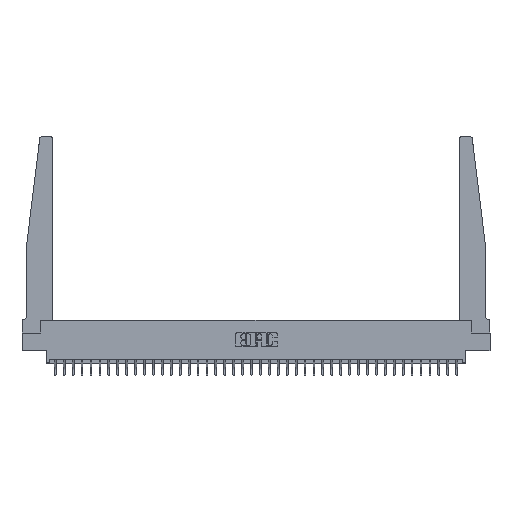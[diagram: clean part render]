
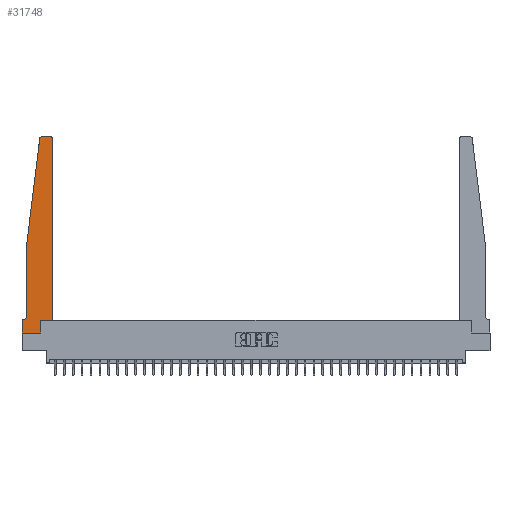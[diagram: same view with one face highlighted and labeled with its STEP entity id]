
A CAD part, top view. The second image highlights one B-rep face of the part: STEP entity #31748.
In plain terms, the highlighted planar face has unit normal (0, 0, 1).
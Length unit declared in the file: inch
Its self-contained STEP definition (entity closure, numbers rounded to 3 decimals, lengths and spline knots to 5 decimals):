
#67 = DIRECTION ( 'NONE',  ( 0., 0., 1. ) ) ;
#528 = VERTEX_POINT ( 'NONE', #5007 ) ;
#725 = CARTESIAN_POINT ( 'NONE',  ( 0.065, 0.2375, 0.37 ) ) ;
#1007 = DIRECTION ( 'NONE',  ( 0., -1., 0. ) ) ;
#2030 = ORIENTED_EDGE ( 'NONE', *, *, #10077, .T. ) ;
#2631 = VERTEX_POINT ( 'NONE', #725 ) ;
#2640 = VECTOR ( 'NONE', #1007, 39.37008 ) ;
#2778 = DIRECTION ( 'NONE',  ( 0., 0., -1. ) ) ;
#3028 = EDGE_CURVE ( 'NONE', #4124, #26963, #29324, .T. ) ;
#3127 = VECTOR ( 'NONE', #14454, 39.37008 ) ;
#3494 = LINE ( 'NONE', #19946, #2640 ) ;
#3542 = CARTESIAN_POINT ( 'NONE',  ( 0.27653, 2.72, 0.37 ) ) ;
#4124 = VERTEX_POINT ( 'NONE', #23718 ) ;
#4164 = ORIENTED_EDGE ( 'NONE', *, *, #18975, .T. ) ;
#4481 = VECTOR ( 'NONE', #12872, 39.37008 ) ;
#4865 = CARTESIAN_POINT ( 'NONE',  ( 0.425, 2.72, 0.37 ) ) ;
#5007 = CARTESIAN_POINT ( 'NONE',  ( 0., 0.1875, 0.37 ) ) ;
#5064 = DIRECTION ( 'NONE',  ( 0., -1., 0. ) ) ;
#5184 = VECTOR ( 'NONE', #30541, 39.37008 ) ;
#5293 = CARTESIAN_POINT ( 'NONE',  ( 0.015, 0.1875, 0.37 ) ) ;
#5635 = CARTESIAN_POINT ( 'NONE',  ( 0.425, 0.18, 0.37 ) ) ;
#6027 = VERTEX_POINT ( 'NONE', #22489 ) ;
#6119 = CARTESIAN_POINT ( 'NONE',  ( 0.2605, 0.18, 0.37 ) ) ;
#6296 = DIRECTION ( 'NONE',  ( 1., 0., 0. ) ) ;
#6726 = ORIENTED_EDGE ( 'NONE', *, *, #7844, .T. ) ;
#7589 = EDGE_CURVE ( 'NONE', #21215, #4124, #32333, .T. ) ;
#7811 = CARTESIAN_POINT ( 'NONE',  ( 0.065, 1.25, 0.37 ) ) ;
#7844 = EDGE_CURVE ( 'NONE', #528, #31717, #3494, .T. ) ;
#8389 = DIRECTION ( 'NONE',  ( 1., 0., 0. ) ) ;
#8815 = VECTOR ( 'NONE', #8389, 39.37008 ) ;
#9297 = ORIENTED_EDGE ( 'NONE', *, *, #11489, .T. ) ;
#9444 = PLANE ( 'NONE',  #27056 ) ;
#9688 = EDGE_CURVE ( 'NONE', #26963, #18637, #15705, .T. ) ;
#10077 = EDGE_CURVE ( 'NONE', #6027, #2631, #18207, .T. ) ;
#10112 = ORIENTED_EDGE ( 'NONE', *, *, #9688, .T. ) ;
#10209 = EDGE_LOOP ( 'NONE', ( #24317, #10112, #9297, #2030, #22724, #21066, #6726, #18561, #4164, #30090, #34571, #20601 ) ) ;
#11489 = EDGE_CURVE ( 'NONE', #18637, #6027, #33758, .T. ) ;
#12085 = LINE ( 'NONE', #19870, #3127 ) ;
#12145 = DIRECTION ( 'NONE',  ( 0., 0., 1. ) ) ;
#12872 = DIRECTION ( 'NONE',  ( -1., 0., 0. ) ) ;
#14005 = EDGE_CURVE ( 'NONE', #23192, #21215, #12085, .T. ) ;
#14454 = DIRECTION ( 'NONE',  ( 0., 1., 0. ) ) ;
#14543 = CARTESIAN_POINT ( 'NONE',  ( 0., 0., 0.37 ) ) ;
#15163 = CARTESIAN_POINT ( 'NONE',  ( 0.2605, 0., 0.37 ) ) ;
#15474 = CARTESIAN_POINT ( 'NONE',  ( 0.425, 0.18, 0.37 ) ) ;
#15544 = DIRECTION ( 'NONE',  ( -1., 0., 0. ) ) ;
#15705 = CIRCLE ( 'NONE', #33388, 0.03 ) ;
#16103 = VECTOR ( 'NONE', #15544, 39.37008 ) ;
#16344 = CARTESIAN_POINT ( 'NONE',  ( 0.395, 2.72, 0.37 ) ) ;
#16858 = CARTESIAN_POINT ( 'NONE',  ( 0.2605, 0.18, 0.37 ) ) ;
#18207 = LINE ( 'NONE', #7811, #31375 ) ;
#18561 = ORIENTED_EDGE ( 'NONE', *, *, #33113, .T. ) ;
#18637 = VERTEX_POINT ( 'NONE', #28926 ) ;
#18883 = LINE ( 'NONE', #28682, #4481 ) ;
#18975 = EDGE_CURVE ( 'NONE', #19804, #21475, #21946, .T. ) ;
#19022 = CARTESIAN_POINT ( 'NONE',  ( 0.015, 0.2375, 0.37 ) ) ;
#19043 = DIRECTION ( 'NONE',  ( 1., 0., 0. ) ) ;
#19045 = AXIS2_PLACEMENT_3D ( 'NONE', #16344, #67, #19043 ) ;
#19773 = VECTOR ( 'NONE', #22805, 39.37008 ) ;
#19804 = VERTEX_POINT ( 'NONE', #15163 ) ;
#19870 = CARTESIAN_POINT ( 'NONE',  ( 0.425, 0.18, 0.37 ) ) ;
#19946 = CARTESIAN_POINT ( 'NONE',  ( 0., 0., 0.37 ) ) ;
#20601 = ORIENTED_EDGE ( 'NONE', *, *, #7589, .T. ) ;
#20924 = CARTESIAN_POINT ( 'NONE',  ( 0.25, 2.75, 0.37 ) ) ;
#21066 = ORIENTED_EDGE ( 'NONE', *, *, #31259, .T. ) ;
#21215 = VERTEX_POINT ( 'NONE', #4865 ) ;
#21475 = VERTEX_POINT ( 'NONE', #16858 ) ;
#21687 = DIRECTION ( 'NONE',  ( -1., 0., 0. ) ) ;
#21946 = LINE ( 'NONE', #6119, #28096 ) ;
#22412 = DIRECTION ( 'NONE',  ( 0., 0., 1. ) ) ;
#22489 = CARTESIAN_POINT ( 'NONE',  ( 0.065, 1.25, 0.37 ) ) ;
#22724 = ORIENTED_EDGE ( 'NONE', *, *, #29507, .T. ) ;
#22805 = DIRECTION ( 'NONE',  ( -0.122, -0.992, 0. ) ) ;
#23192 = VERTEX_POINT ( 'NONE', #15474 ) ;
#23634 = AXIS2_PLACEMENT_3D ( 'NONE', #19022, #2778, #21687 ) ;
#23718 = CARTESIAN_POINT ( 'NONE',  ( 0.395, 2.75, 0.37 ) ) ;
#24317 = ORIENTED_EDGE ( 'NONE', *, *, #3028, .T. ) ;
#26574 = LINE ( 'NONE', #14543, #5184 ) ;
#26963 = VERTEX_POINT ( 'NONE', #33178 ) ;
#27056 = AXIS2_PLACEMENT_3D ( 'NONE', #28080, #12145, #30721 ) ;
#27350 = VERTEX_POINT ( 'NONE', #5293 ) ;
#27522 = DIRECTION ( 'NONE',  ( 0., 1., 0. ) ) ;
#28080 = CARTESIAN_POINT ( 'NONE',  ( 0., 0.1875, 0.37 ) ) ;
#28096 = VECTOR ( 'NONE', #27522, 39.37008 ) ;
#28682 = CARTESIAN_POINT ( 'NONE',  ( 0.065, 0.1875, 0.37 ) ) ;
#28926 = CARTESIAN_POINT ( 'NONE',  ( 0.24675, 2.72367, 0.37 ) ) ;
#29324 = LINE ( 'NONE', #20924, #16103 ) ;
#29507 = EDGE_CURVE ( 'NONE', #2631, #27350, #30891, .T. ) ;
#29561 = EDGE_CURVE ( 'NONE', #21475, #23192, #30059, .T. ) ;
#30059 = LINE ( 'NONE', #5635, #8815 ) ;
#30090 = ORIENTED_EDGE ( 'NONE', *, *, #29561, .T. ) ;
#30541 = DIRECTION ( 'NONE',  ( 1., 0., 0. ) ) ;
#30712 = CARTESIAN_POINT ( 'NONE',  ( 0.065, 1.25, 0.37 ) ) ;
#30721 = DIRECTION ( 'NONE',  ( 1., 0., 0. ) ) ;
#30891 = CIRCLE ( 'NONE', #23634, 0.05 ) ;
#31259 = EDGE_CURVE ( 'NONE', #27350, #528, #18883, .T. ) ;
#31375 = VECTOR ( 'NONE', #5064, 39.37008 ) ;
#31717 = VERTEX_POINT ( 'NONE', #33240 ) ;
#31748 = ADVANCED_FACE ( 'NONE', ( #32824 ), #9444, .T. ) ;
#32333 = CIRCLE ( 'NONE', #19045, 0.03 ) ;
#32824 = FACE_OUTER_BOUND ( 'NONE', #10209, .T. ) ;
#33113 = EDGE_CURVE ( 'NONE', #31717, #19804, #26574, .T. ) ;
#33178 = CARTESIAN_POINT ( 'NONE',  ( 0.27653, 2.75, 0.37 ) ) ;
#33240 = CARTESIAN_POINT ( 'NONE',  ( 0., 0., 0.37 ) ) ;
#33388 = AXIS2_PLACEMENT_3D ( 'NONE', #3542, #22412, #6296 ) ;
#33758 = LINE ( 'NONE', #30712, #19773 ) ;
#34571 = ORIENTED_EDGE ( 'NONE', *, *, #14005, .T. ) ;
